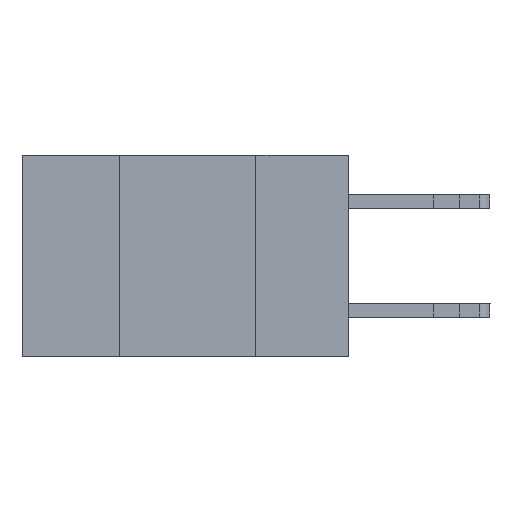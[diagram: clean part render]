
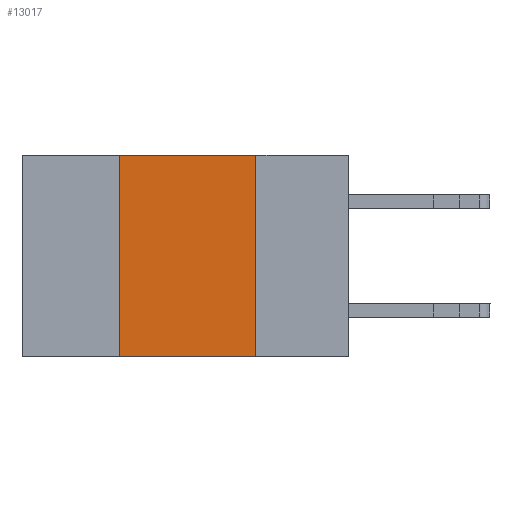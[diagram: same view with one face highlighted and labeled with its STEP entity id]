
A CAD part, left-side view. The second image highlights one B-rep face of the part: STEP entity #13017.
In plain terms, the highlighted planar face has unit normal (-1, 0, 0).
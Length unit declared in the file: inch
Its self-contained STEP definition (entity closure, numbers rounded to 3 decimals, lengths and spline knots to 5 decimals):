
#85 = LINE ( 'NONE', #23692, #3468 ) ;
#838 = VECTOR ( 'NONE', #16362, 39.37008 ) ;
#1207 = VERTEX_POINT ( 'NONE', #10730 ) ;
#2342 = ORIENTED_EDGE ( 'NONE', *, *, #10071, .F. ) ;
#2560 = ORIENTED_EDGE ( 'NONE', *, *, #16296, .F. ) ;
#3468 = VECTOR ( 'NONE', #10612, 39.37008 ) ;
#4457 = VERTEX_POINT ( 'NONE', #18311 ) ;
#5505 = DIRECTION ( 'NONE',  ( 1., 0., 0. ) ) ;
#7974 = LINE ( 'NONE', #8781, #16590 ) ;
#8781 = CARTESIAN_POINT ( 'NONE',  ( 0., 0.42, 0. ) ) ;
#10071 = EDGE_CURVE ( 'NONE', #1207, #12609, #22511, .T. ) ;
#10612 = DIRECTION ( 'NONE',  ( 0., -1., 0. ) ) ;
#10730 = CARTESIAN_POINT ( 'NONE',  ( 0., 0.17, 0. ) ) ;
#11154 = EDGE_CURVE ( 'NONE', #4457, #23757, #7974, .T. ) ;
#12609 = VERTEX_POINT ( 'NONE', #14976 ) ;
#12994 = ORIENTED_EDGE ( 'NONE', *, *, #21107, .T. ) ;
#13017 = ADVANCED_FACE ( 'NONE', ( #25126 ), #17332, .F. ) ;
#13286 = DIRECTION ( 'NONE',  ( 0., 0., -1. ) ) ;
#14976 = CARTESIAN_POINT ( 'NONE',  ( 0., 0.17, -0.37 ) ) ;
#15202 = EDGE_LOOP ( 'NONE', ( #2342, #2560, #20441, #12994 ) ) ;
#16296 = EDGE_CURVE ( 'NONE', #23757, #1207, #85, .T. ) ;
#16362 = DIRECTION ( 'NONE',  ( 0., -1., 0. ) ) ;
#16590 = VECTOR ( 'NONE', #24700, 39.37008 ) ;
#17332 = PLANE ( 'NONE',  #22836 ) ;
#18311 = CARTESIAN_POINT ( 'NONE',  ( 0., 0.42, -0.37 ) ) ;
#18333 = CARTESIAN_POINT ( 'NONE',  ( 0., 0.6, -0.37 ) ) ;
#19223 = CARTESIAN_POINT ( 'NONE',  ( 0., 0.6, 0. ) ) ;
#20023 = CARTESIAN_POINT ( 'NONE',  ( 0., 0.17, 0. ) ) ;
#20441 = ORIENTED_EDGE ( 'NONE', *, *, #11154, .F. ) ;
#21107 = EDGE_CURVE ( 'NONE', #4457, #12609, #23631, .T. ) ;
#22511 = LINE ( 'NONE', #20023, #24702 ) ;
#22836 = AXIS2_PLACEMENT_3D ( 'NONE', #19223, #5505, #13286 ) ;
#23631 = LINE ( 'NONE', #18333, #838 ) ;
#23692 = CARTESIAN_POINT ( 'NONE',  ( 0., 0.6, 0. ) ) ;
#23757 = VERTEX_POINT ( 'NONE', #24311 ) ;
#24005 = DIRECTION ( 'NONE',  ( 0., 0., -1. ) ) ;
#24311 = CARTESIAN_POINT ( 'NONE',  ( 0., 0.42, 0. ) ) ;
#24700 = DIRECTION ( 'NONE',  ( 0., 0., 1. ) ) ;
#24702 = VECTOR ( 'NONE', #24005, 39.37008 ) ;
#25126 = FACE_OUTER_BOUND ( 'NONE', #15202, .T. ) ;
